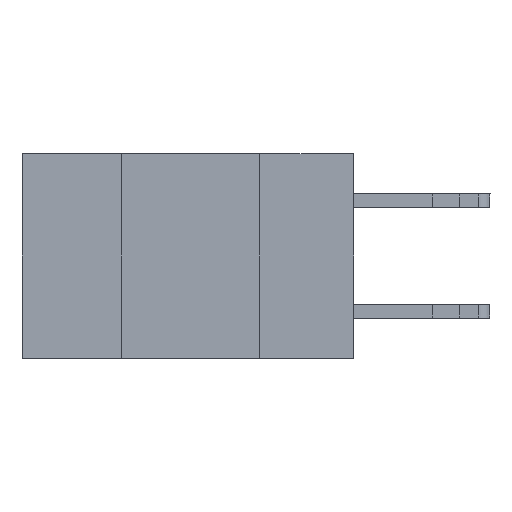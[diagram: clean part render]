
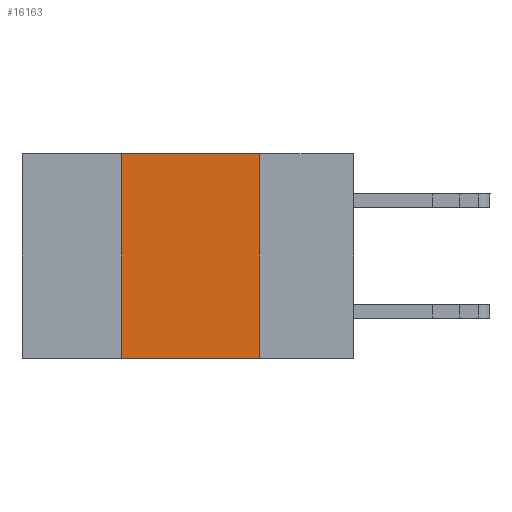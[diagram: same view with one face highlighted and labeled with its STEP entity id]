
A CAD part, left-side view. The second image highlights one B-rep face of the part: STEP entity #16163.
In plain terms, the highlighted planar face has unit normal (-1, 0, 0).
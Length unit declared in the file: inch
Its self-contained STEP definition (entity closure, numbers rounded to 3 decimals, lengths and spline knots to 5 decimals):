
#839 = CARTESIAN_POINT ( 'NONE',  ( 0., 0.42, 0. ) ) ;
#1168 = PLANE ( 'NONE',  #26179 ) ;
#1634 = DIRECTION ( 'NONE',  ( 0., -1., 0. ) ) ;
#1665 = CARTESIAN_POINT ( 'NONE',  ( 0., 0.17, -0.37 ) ) ;
#2220 = ORIENTED_EDGE ( 'NONE', *, *, #14080, .T. ) ;
#2487 = CARTESIAN_POINT ( 'NONE',  ( 0., 0.42, 0. ) ) ;
#3055 = ORIENTED_EDGE ( 'NONE', *, *, #32131, .F. ) ;
#4691 = VERTEX_POINT ( 'NONE', #1665 ) ;
#5120 = VECTOR ( 'NONE', #24476, 39.37008 ) ;
#6221 = VERTEX_POINT ( 'NONE', #8891 ) ;
#6768 = CARTESIAN_POINT ( 'NONE',  ( 0., 0.6, -0.37 ) ) ;
#8891 = CARTESIAN_POINT ( 'NONE',  ( 0., 0.42, -0.37 ) ) ;
#9604 = ORIENTED_EDGE ( 'NONE', *, *, #20265, .F. ) ;
#9892 = CARTESIAN_POINT ( 'NONE',  ( 0., 0.6, 0. ) ) ;
#10158 = EDGE_CURVE ( 'NONE', #18284, #4691, #15469, .T. ) ;
#10528 = VECTOR ( 'NONE', #1634, 39.37008 ) ;
#11809 = DIRECTION ( 'NONE',  ( 0., 0., -1. ) ) ;
#11998 = VECTOR ( 'NONE', #12496, 39.37008 ) ;
#12496 = DIRECTION ( 'NONE',  ( 0., -1., 0. ) ) ;
#12971 = FACE_OUTER_BOUND ( 'NONE', #20529, .T. ) ;
#14080 = EDGE_CURVE ( 'NONE', #6221, #4691, #31299, .T. ) ;
#14840 = LINE ( 'NONE', #2487, #5120 ) ;
#15469 = LINE ( 'NONE', #25899, #20176 ) ;
#16163 = ADVANCED_FACE ( 'NONE', ( #12971 ), #1168, .F. ) ;
#16735 = VERTEX_POINT ( 'NONE', #839 ) ;
#18284 = VERTEX_POINT ( 'NONE', #21722 ) ;
#20176 = VECTOR ( 'NONE', #30948, 39.37008 ) ;
#20265 = EDGE_CURVE ( 'NONE', #16735, #18284, #21800, .T. ) ;
#20529 = EDGE_LOOP ( 'NONE', ( #29050, #9604, #3055, #2220 ) ) ;
#21656 = DIRECTION ( 'NONE',  ( 1., 0., 0. ) ) ;
#21722 = CARTESIAN_POINT ( 'NONE',  ( 0., 0.17, 0. ) ) ;
#21800 = LINE ( 'NONE', #9892, #11998 ) ;
#24138 = CARTESIAN_POINT ( 'NONE',  ( 0., 0.6, 0. ) ) ;
#24476 = DIRECTION ( 'NONE',  ( 0., 0., 1. ) ) ;
#25899 = CARTESIAN_POINT ( 'NONE',  ( 0., 0.17, 0. ) ) ;
#26179 = AXIS2_PLACEMENT_3D ( 'NONE', #24138, #21656, #11809 ) ;
#29050 = ORIENTED_EDGE ( 'NONE', *, *, #10158, .F. ) ;
#30948 = DIRECTION ( 'NONE',  ( 0., 0., -1. ) ) ;
#31299 = LINE ( 'NONE', #6768, #10528 ) ;
#32131 = EDGE_CURVE ( 'NONE', #6221, #16735, #14840, .T. ) ;
